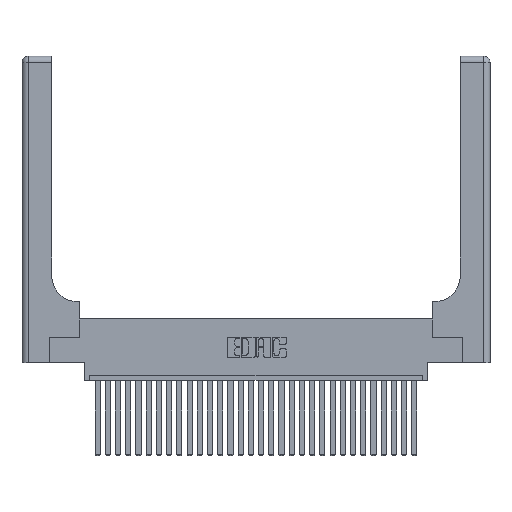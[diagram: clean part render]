
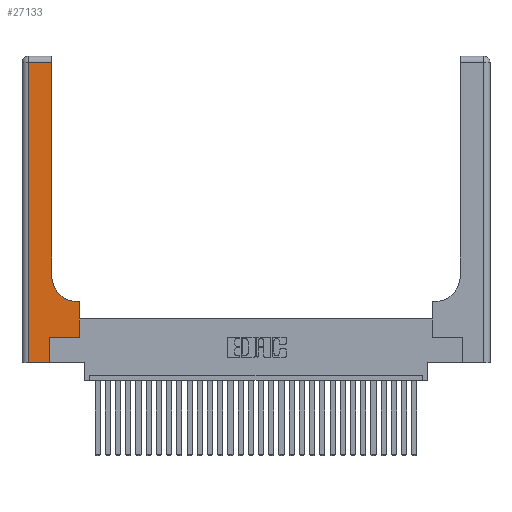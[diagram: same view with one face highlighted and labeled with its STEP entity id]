
A CAD part, top view. The second image highlights one B-rep face of the part: STEP entity #27133.
In plain terms, the highlighted planar face has unit normal (0, 0, 1).
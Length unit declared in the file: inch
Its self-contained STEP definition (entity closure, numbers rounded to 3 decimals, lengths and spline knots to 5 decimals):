
#219 = VECTOR ( 'NONE', #6228, 39.37008 ) ;
#586 = VERTEX_POINT ( 'NONE', #2307 ) ;
#624 = LINE ( 'NONE', #13606, #19447 ) ;
#969 = LINE ( 'NONE', #4458, #18301 ) ;
#1092 = VERTEX_POINT ( 'NONE', #4715 ) ;
#1414 = CARTESIAN_POINT ( 'NONE',  ( 0., 3., 0.37 ) ) ;
#1986 = EDGE_CURVE ( 'NONE', #9094, #24027, #624, .T. ) ;
#2260 = VERTEX_POINT ( 'NONE', #13145 ) ;
#2307 = CARTESIAN_POINT ( 'NONE',  ( 0.5415, 0.6, 0.37 ) ) ;
#2512 = EDGE_CURVE ( 'NONE', #24027, #586, #969, .T. ) ;
#3683 = PLANE ( 'NONE',  #8924 ) ;
#3758 = ORIENTED_EDGE ( 'NONE', *, *, #17009, .T. ) ;
#4133 = ORIENTED_EDGE ( 'NONE', *, *, #10507, .T. ) ;
#4458 = CARTESIAN_POINT ( 'NONE',  ( 0.2915, 0.6, 0.37 ) ) ;
#4715 = CARTESIAN_POINT ( 'NONE',  ( 0.2915, 0.85, 0.37 ) ) ;
#4902 = EDGE_LOOP ( 'NONE', ( #3758, #25731, #4133, #10691, #18194, #15553, #19125, #17566, #5802 ) ) ;
#5138 = CIRCLE ( 'NONE', #21745, 0.25 ) ;
#5199 = DIRECTION ( 'NONE',  ( -1., 0., 0. ) ) ;
#5802 = ORIENTED_EDGE ( 'NONE', *, *, #24212, .T. ) ;
#6228 = DIRECTION ( 'NONE',  ( 0., 1., 0. ) ) ;
#6271 = DIRECTION ( 'NONE',  ( 0., 1., 0. ) ) ;
#6928 = DIRECTION ( 'NONE',  ( -1., 0., 0. ) ) ;
#8266 = VERTEX_POINT ( 'NONE', #13180 ) ;
#8924 = AXIS2_PLACEMENT_3D ( 'NONE', #1414, #17936, #24714 ) ;
#9059 = EDGE_CURVE ( 'NONE', #21724, #19595, #10248, .T. ) ;
#9094 = VERTEX_POINT ( 'NONE', #29120 ) ;
#9213 = DIRECTION ( 'NONE',  ( 0., 0., -1. ) ) ;
#9225 = VECTOR ( 'NONE', #24427, 39.37008 ) ;
#9841 = CARTESIAN_POINT ( 'NONE',  ( 0., 2.94, 0.37 ) ) ;
#10248 = LINE ( 'NONE', #9841, #27616 ) ;
#10507 = EDGE_CURVE ( 'NONE', #19595, #2260, #19906, .T. ) ;
#10691 = ORIENTED_EDGE ( 'NONE', *, *, #25397, .T. ) ;
#12386 = EDGE_CURVE ( 'NONE', #13506, #8266, #14566, .T. ) ;
#13145 = CARTESIAN_POINT ( 'NONE',  ( 0.06, 0., 0.37 ) ) ;
#13180 = CARTESIAN_POINT ( 'NONE',  ( 0.269, 0.25, 0.37 ) ) ;
#13506 = VERTEX_POINT ( 'NONE', #29670 ) ;
#13606 = CARTESIAN_POINT ( 'NONE',  ( 0.5585, 0.25, 0.37 ) ) ;
#14019 = CARTESIAN_POINT ( 'NONE',  ( 0.2915, 3., 0.37 ) ) ;
#14566 = LINE ( 'NONE', #20398, #219 ) ;
#14779 = DIRECTION ( 'NONE',  ( 0., -1., 0. ) ) ;
#15553 = ORIENTED_EDGE ( 'NONE', *, *, #17269, .T. ) ;
#17009 = EDGE_CURVE ( 'NONE', #1092, #21724, #25131, .T. ) ;
#17269 = EDGE_CURVE ( 'NONE', #8266, #9094, #18118, .T. ) ;
#17566 = ORIENTED_EDGE ( 'NONE', *, *, #2512, .T. ) ;
#17936 = DIRECTION ( 'NONE',  ( 0., 0., -1. ) ) ;
#18118 = LINE ( 'NONE', #26703, #9225 ) ;
#18145 = VECTOR ( 'NONE', #25470, 39.37008 ) ;
#18194 = ORIENTED_EDGE ( 'NONE', *, *, #12386, .T. ) ;
#18301 = VECTOR ( 'NONE', #6928, 39.37008 ) ;
#18947 = DIRECTION ( 'NONE',  ( 1., 0., 0. ) ) ;
#19125 = ORIENTED_EDGE ( 'NONE', *, *, #1986, .T. ) ;
#19447 = VECTOR ( 'NONE', #6271, 39.37008 ) ;
#19595 = VERTEX_POINT ( 'NONE', #25083 ) ;
#19906 = LINE ( 'NONE', #30402, #26496 ) ;
#20276 = VECTOR ( 'NONE', #18947, 39.37008 ) ;
#20398 = CARTESIAN_POINT ( 'NONE',  ( 0.269, 0., 0.37 ) ) ;
#21119 = DIRECTION ( 'NONE',  ( 1., 0., 0. ) ) ;
#21226 = CARTESIAN_POINT ( 'NONE',  ( 0., 0., 0.37 ) ) ;
#21724 = VERTEX_POINT ( 'NONE', #26205 ) ;
#21745 = AXIS2_PLACEMENT_3D ( 'NONE', #23487, #9213, #21119 ) ;
#22043 = FACE_OUTER_BOUND ( 'NONE', #4902, .T. ) ;
#22407 = CARTESIAN_POINT ( 'NONE',  ( 0.5585, 0.6, 0.37 ) ) ;
#23487 = CARTESIAN_POINT ( 'NONE',  ( 0.5415, 0.85, 0.37 ) ) ;
#24027 = VERTEX_POINT ( 'NONE', #22407 ) ;
#24212 = EDGE_CURVE ( 'NONE', #586, #1092, #5138, .T. ) ;
#24427 = DIRECTION ( 'NONE',  ( 1., 0., 0. ) ) ;
#24714 = DIRECTION ( 'NONE',  ( -1., 0., 0. ) ) ;
#25083 = CARTESIAN_POINT ( 'NONE',  ( 0.06, 2.94, 0.37 ) ) ;
#25131 = LINE ( 'NONE', #14019, #18145 ) ;
#25397 = EDGE_CURVE ( 'NONE', #2260, #13506, #27281, .T. ) ;
#25470 = DIRECTION ( 'NONE',  ( 0., 1., 0. ) ) ;
#25731 = ORIENTED_EDGE ( 'NONE', *, *, #9059, .T. ) ;
#26205 = CARTESIAN_POINT ( 'NONE',  ( 0.2915, 2.94, 0.37 ) ) ;
#26496 = VECTOR ( 'NONE', #14779, 39.37008 ) ;
#26703 = CARTESIAN_POINT ( 'NONE',  ( 0.269, 0.25, 0.37 ) ) ;
#27133 = ADVANCED_FACE ( 'NONE', ( #22043 ), #3683, .F. ) ;
#27281 = LINE ( 'NONE', #21226, #20276 ) ;
#27616 = VECTOR ( 'NONE', #5199, 39.37008 ) ;
#29120 = CARTESIAN_POINT ( 'NONE',  ( 0.5585, 0.25, 0.37 ) ) ;
#29670 = CARTESIAN_POINT ( 'NONE',  ( 0.269, 0., 0.37 ) ) ;
#30402 = CARTESIAN_POINT ( 'NONE',  ( 0.06, 3., 0.37 ) ) ;
